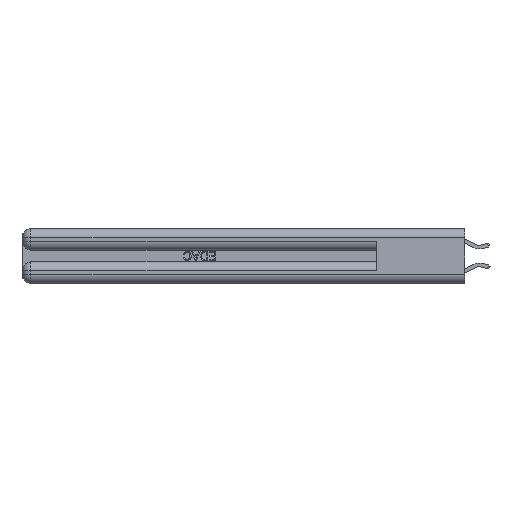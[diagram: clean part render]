
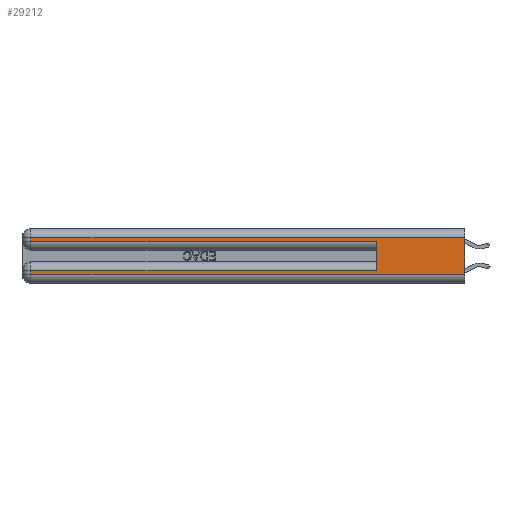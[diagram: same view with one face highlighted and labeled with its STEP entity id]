
A CAD part, left-side view. The second image highlights one B-rep face of the part: STEP entity #29212.
In plain terms, the highlighted planar face has unit normal (-1, 0, 0).
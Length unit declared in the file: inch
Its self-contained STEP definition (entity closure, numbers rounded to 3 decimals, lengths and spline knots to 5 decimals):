
#576 = CARTESIAN_POINT ( 'NONE',  ( 0., 2.94, 0.37 ) ) ;
#833 = EDGE_LOOP ( 'NONE', ( #2710, #24867, #23699, #12602, #20357, #21659, #9911, #12541 ) ) ;
#1529 = CARTESIAN_POINT ( 'NONE',  ( 0., 0., 0.085 ) ) ;
#2215 = FACE_OUTER_BOUND ( 'NONE', #833, .T. ) ;
#2359 = DIRECTION ( 'NONE',  ( 1., 0., 0. ) ) ;
#2710 = ORIENTED_EDGE ( 'NONE', *, *, #14210, .F. ) ;
#3279 = CARTESIAN_POINT ( 'NONE',  ( 0., 0.6, 0.085 ) ) ;
#3445 = VECTOR ( 'NONE', #15953, 39.37008 ) ;
#3598 = VERTEX_POINT ( 'NONE', #10252 ) ;
#4093 = DIRECTION ( 'NONE',  ( 0., 1., 0. ) ) ;
#4171 = VECTOR ( 'NONE', #4093, 39.37008 ) ;
#4653 = CARTESIAN_POINT ( 'NONE',  ( 0., 0., 0.31 ) ) ;
#5605 = LINE ( 'NONE', #15413, #25014 ) ;
#5974 = LINE ( 'NONE', #6150, #3445 ) ;
#6150 = CARTESIAN_POINT ( 'NONE',  ( 0., 0., 0.37 ) ) ;
#7456 = DIRECTION ( 'NONE',  ( 0., 0., -1. ) ) ;
#7497 = CARTESIAN_POINT ( 'NONE',  ( 0., 0., 0.285 ) ) ;
#8076 = EDGE_CURVE ( 'NONE', #28532, #22892, #19051, .T. ) ;
#9035 = EDGE_CURVE ( 'NONE', #10490, #27980, #27732, .T. ) ;
#9768 = CARTESIAN_POINT ( 'NONE',  ( 0., 0., 0.37 ) ) ;
#9911 = ORIENTED_EDGE ( 'NONE', *, *, #19226, .T. ) ;
#10252 = CARTESIAN_POINT ( 'NONE',  ( 0., 0., 0.31 ) ) ;
#10490 = VERTEX_POINT ( 'NONE', #27105 ) ;
#11291 = VECTOR ( 'NONE', #7456, 39.37008 ) ;
#12482 = DIRECTION ( 'NONE',  ( 0., 0., -1. ) ) ;
#12541 = ORIENTED_EDGE ( 'NONE', *, *, #9035, .T. ) ;
#12602 = ORIENTED_EDGE ( 'NONE', *, *, #19897, .T. ) ;
#14210 = EDGE_CURVE ( 'NONE', #3598, #27980, #5974, .T. ) ;
#14518 = CARTESIAN_POINT ( 'NONE',  ( 0., 0.6, 0.145 ) ) ;
#14907 = LINE ( 'NONE', #4653, #31316 ) ;
#15413 = CARTESIAN_POINT ( 'NONE',  ( 0., 2.94, 0.37 ) ) ;
#15953 = DIRECTION ( 'NONE',  ( 0., 0., -1. ) ) ;
#17291 = DIRECTION ( 'NONE',  ( 0., -1., 0. ) ) ;
#17458 = VECTOR ( 'NONE', #17291, 39.37008 ) ;
#19051 = LINE ( 'NONE', #14518, #29703 ) ;
#19226 = EDGE_CURVE ( 'NONE', #19649, #10490, #22562, .T. ) ;
#19649 = VERTEX_POINT ( 'NONE', #27193 ) ;
#19874 = EDGE_CURVE ( 'NONE', #3598, #27776, #14907, .T. ) ;
#19897 = EDGE_CURVE ( 'NONE', #27769, #22892, #31594, .T. ) ;
#20038 = CARTESIAN_POINT ( 'NONE',  ( 0., 0., 0.06 ) ) ;
#20357 = ORIENTED_EDGE ( 'NONE', *, *, #8076, .F. ) ;
#20831 = DIRECTION ( 'NONE',  ( 0., 0., -1. ) ) ;
#20957 = LINE ( 'NONE', #1529, #4171 ) ;
#21659 = ORIENTED_EDGE ( 'NONE', *, *, #28704, .T. ) ;
#22562 = LINE ( 'NONE', #576, #11291 ) ;
#22892 = VERTEX_POINT ( 'NONE', #26698 ) ;
#23282 = VECTOR ( 'NONE', #27883, 39.37008 ) ;
#23699 = ORIENTED_EDGE ( 'NONE', *, *, #30662, .T. ) ;
#24214 = CARTESIAN_POINT ( 'NONE',  ( 0., 2.94, 0.285 ) ) ;
#24867 = ORIENTED_EDGE ( 'NONE', *, *, #19874, .T. ) ;
#25001 = PLANE ( 'NONE',  #27510 ) ;
#25014 = VECTOR ( 'NONE', #20831, 39.37008 ) ;
#26319 = CARTESIAN_POINT ( 'NONE',  ( 0., 2.94, 0.31 ) ) ;
#26422 = DIRECTION ( 'NONE',  ( 0., 0., 1. ) ) ;
#26698 = CARTESIAN_POINT ( 'NONE',  ( 0., 0.6, 0.285 ) ) ;
#26818 = CARTESIAN_POINT ( 'NONE',  ( 0., 0., 0.06 ) ) ;
#27105 = CARTESIAN_POINT ( 'NONE',  ( 0., 2.94, 0.06 ) ) ;
#27193 = CARTESIAN_POINT ( 'NONE',  ( 0., 2.94, 0.085 ) ) ;
#27510 = AXIS2_PLACEMENT_3D ( 'NONE', #9768, #2359, #12482 ) ;
#27732 = LINE ( 'NONE', #26818, #23282 ) ;
#27769 = VERTEX_POINT ( 'NONE', #24214 ) ;
#27776 = VERTEX_POINT ( 'NONE', #26319 ) ;
#27883 = DIRECTION ( 'NONE',  ( 0., -1., 0. ) ) ;
#27980 = VERTEX_POINT ( 'NONE', #20038 ) ;
#28532 = VERTEX_POINT ( 'NONE', #3279 ) ;
#28704 = EDGE_CURVE ( 'NONE', #28532, #19649, #20957, .T. ) ;
#29212 = ADVANCED_FACE ( 'NONE', ( #2215 ), #25001, .F. ) ;
#29517 = DIRECTION ( 'NONE',  ( 0., 1., 0. ) ) ;
#29703 = VECTOR ( 'NONE', #26422, 39.37008 ) ;
#30662 = EDGE_CURVE ( 'NONE', #27776, #27769, #5605, .T. ) ;
#31316 = VECTOR ( 'NONE', #29517, 39.37008 ) ;
#31594 = LINE ( 'NONE', #7497, #17458 ) ;
